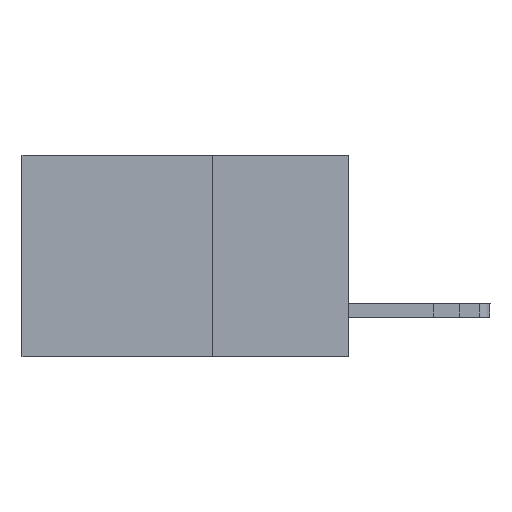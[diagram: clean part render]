
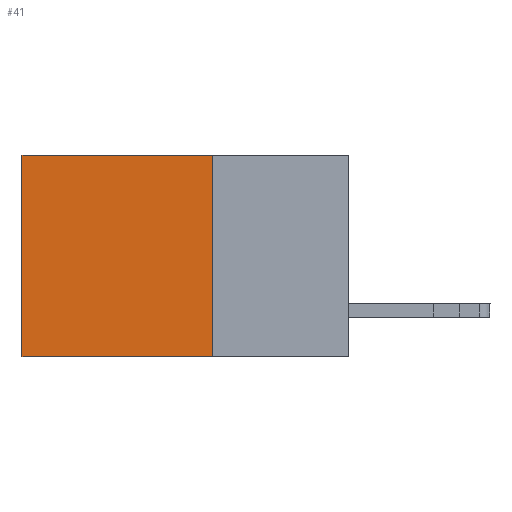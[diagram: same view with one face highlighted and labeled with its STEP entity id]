
A CAD part, left-side view. The second image highlights one B-rep face of the part: STEP entity #41.
In plain terms, the highlighted planar face has unit normal (-1, 0, 0).
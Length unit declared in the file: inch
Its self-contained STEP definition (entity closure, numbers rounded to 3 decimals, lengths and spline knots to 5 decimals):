
#41 = ADVANCED_FACE ( 'NONE', ( #3380 ), #12180, .F. ) ;
#438 = CARTESIAN_POINT ( 'NONE',  ( 0.2615, 0.25, -0.37 ) ) ;
#591 = LINE ( 'NONE', #6665, #11528 ) ;
#2058 = VERTEX_POINT ( 'NONE', #8374 ) ;
#2287 = VECTOR ( 'NONE', #6818, 39.37008 ) ;
#2617 = LINE ( 'NONE', #2705, #9488 ) ;
#2705 = CARTESIAN_POINT ( 'NONE',  ( 0.2615, 0.25, -0.37 ) ) ;
#3380 = FACE_OUTER_BOUND ( 'NONE', #11578, .T. ) ;
#4029 = CARTESIAN_POINT ( 'NONE',  ( 0.2615, 0.6, -0.37 ) ) ;
#4326 = VERTEX_POINT ( 'NONE', #4543 ) ;
#4543 = CARTESIAN_POINT ( 'NONE',  ( 0.2615, 0.25, 0. ) ) ;
#4713 = LINE ( 'NONE', #13703, #15203 ) ;
#5350 = EDGE_CURVE ( 'NONE', #4326, #2058, #591, .T. ) ;
#6665 = CARTESIAN_POINT ( 'NONE',  ( 0.2615, 0.25, 0. ) ) ;
#6807 = AXIS2_PLACEMENT_3D ( 'NONE', #438, #10097, #13431 ) ;
#6818 = DIRECTION ( 'NONE',  ( 0., 0., -1. ) ) ;
#6897 = CARTESIAN_POINT ( 'NONE',  ( 0.2615, 0.6, -0.37 ) ) ;
#8177 = VERTEX_POINT ( 'NONE', #6897 ) ;
#8374 = CARTESIAN_POINT ( 'NONE',  ( 0.2615, 0.6, 0. ) ) ;
#9488 = VECTOR ( 'NONE', #12597, 39.37008 ) ;
#9918 = CARTESIAN_POINT ( 'NONE',  ( 0.2615, 0.25, -0.37 ) ) ;
#10097 = DIRECTION ( 'NONE',  ( 1., 0., 0. ) ) ;
#10586 = ORIENTED_EDGE ( 'NONE', *, *, #15082, .F. ) ;
#10607 = EDGE_CURVE ( 'NONE', #2058, #8177, #12819, .T. ) ;
#11528 = VECTOR ( 'NONE', #17561, 39.37008 ) ;
#11578 = EDGE_LOOP ( 'NONE', ( #14788, #11707, #10586, #11704 ) ) ;
#11704 = ORIENTED_EDGE ( 'NONE', *, *, #5350, .T. ) ;
#11707 = ORIENTED_EDGE ( 'NONE', *, *, #16211, .F. ) ;
#12180 = PLANE ( 'NONE',  #6807 ) ;
#12597 = DIRECTION ( 'NONE',  ( 0., 0., -1. ) ) ;
#12819 = LINE ( 'NONE', #4029, #2287 ) ;
#13431 = DIRECTION ( 'NONE',  ( 0., 0., -1. ) ) ;
#13703 = CARTESIAN_POINT ( 'NONE',  ( 0.2615, 0.25, -0.37 ) ) ;
#14788 = ORIENTED_EDGE ( 'NONE', *, *, #10607, .T. ) ;
#15038 = DIRECTION ( 'NONE',  ( 0., 1., 0. ) ) ;
#15082 = EDGE_CURVE ( 'NONE', #4326, #17539, #2617, .T. ) ;
#15203 = VECTOR ( 'NONE', #15038, 39.37008 ) ;
#16211 = EDGE_CURVE ( 'NONE', #17539, #8177, #4713, .T. ) ;
#17539 = VERTEX_POINT ( 'NONE', #9918 ) ;
#17561 = DIRECTION ( 'NONE',  ( 0., 1., 0. ) ) ;
